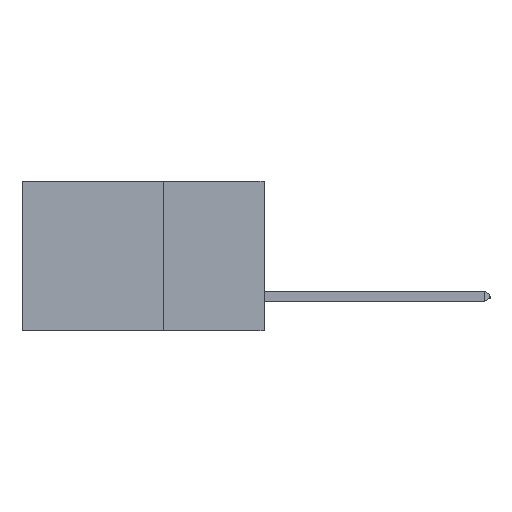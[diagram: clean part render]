
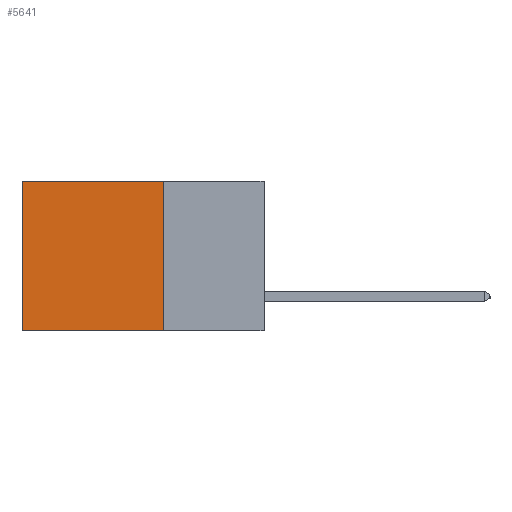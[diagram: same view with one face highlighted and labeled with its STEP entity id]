
A CAD part, left-side view. The second image highlights one B-rep face of the part: STEP entity #5641.
In plain terms, the highlighted planar face has unit normal (-1, 0, 0).
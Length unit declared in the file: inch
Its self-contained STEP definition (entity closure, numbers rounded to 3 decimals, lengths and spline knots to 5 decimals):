
#615 = VECTOR ( 'NONE', #5348, 39.37008 ) ;
#951 = VECTOR ( 'NONE', #5927, 39.37008 ) ;
#1483 = DIRECTION ( 'NONE',  ( 0., 1., 0. ) ) ;
#2137 = EDGE_CURVE ( 'NONE', #5890, #9220, #8862, .T. ) ;
#2466 = CARTESIAN_POINT ( 'NONE',  ( 0.298, 0.25, 0. ) ) ;
#2902 = VERTEX_POINT ( 'NONE', #10271 ) ;
#3218 = DIRECTION ( 'NONE',  ( 0., 0., -1. ) ) ;
#3231 = LINE ( 'NONE', #3879, #5461 ) ;
#3456 = CARTESIAN_POINT ( 'NONE',  ( 0.298, 0.25, 0. ) ) ;
#3628 = LINE ( 'NONE', #6751, #951 ) ;
#3879 = CARTESIAN_POINT ( 'NONE',  ( 0.298, 0.25, -0.37 ) ) ;
#4096 = CARTESIAN_POINT ( 'NONE',  ( 0.298, 0.6, 0. ) ) ;
#5223 = PLANE ( 'NONE',  #7889 ) ;
#5348 = DIRECTION ( 'NONE',  ( 0., 1., 0. ) ) ;
#5354 = DIRECTION ( 'NONE',  ( 1., 0., 0. ) ) ;
#5461 = VECTOR ( 'NONE', #1483, 39.37008 ) ;
#5641 = ADVANCED_FACE ( 'NONE', ( #7710 ), #5223, .F. ) ;
#5890 = VERTEX_POINT ( 'NONE', #2466 ) ;
#5927 = DIRECTION ( 'NONE',  ( 0., 0., -1. ) ) ;
#6011 = VERTEX_POINT ( 'NONE', #8138 ) ;
#6575 = EDGE_CURVE ( 'NONE', #6011, #2902, #3231, .T. ) ;
#6751 = CARTESIAN_POINT ( 'NONE',  ( 0.298, 0.25, 0. ) ) ;
#7211 = EDGE_LOOP ( 'NONE', ( #10741, #10477, #9992, #10467 ) ) ;
#7327 = DIRECTION ( 'NONE',  ( 0., 0., -1. ) ) ;
#7567 = EDGE_CURVE ( 'NONE', #5890, #6011, #3628, .T. ) ;
#7710 = FACE_OUTER_BOUND ( 'NONE', #7211, .T. ) ;
#7889 = AXIS2_PLACEMENT_3D ( 'NONE', #9196, #5354, #7327 ) ;
#8131 = VECTOR ( 'NONE', #3218, 39.37008 ) ;
#8138 = CARTESIAN_POINT ( 'NONE',  ( 0.298, 0.25, -0.37 ) ) ;
#8862 = LINE ( 'NONE', #3456, #615 ) ;
#8937 = CARTESIAN_POINT ( 'NONE',  ( 0.298, 0.6, 0. ) ) ;
#9196 = CARTESIAN_POINT ( 'NONE',  ( 0.298, 0.25, 0. ) ) ;
#9220 = VERTEX_POINT ( 'NONE', #8937 ) ;
#9992 = ORIENTED_EDGE ( 'NONE', *, *, #7567, .F. ) ;
#10271 = CARTESIAN_POINT ( 'NONE',  ( 0.298, 0.6, -0.37 ) ) ;
#10298 = LINE ( 'NONE', #4096, #8131 ) ;
#10467 = ORIENTED_EDGE ( 'NONE', *, *, #2137, .T. ) ;
#10477 = ORIENTED_EDGE ( 'NONE', *, *, #6575, .F. ) ;
#10552 = EDGE_CURVE ( 'NONE', #9220, #2902, #10298, .T. ) ;
#10741 = ORIENTED_EDGE ( 'NONE', *, *, #10552, .T. ) ;
